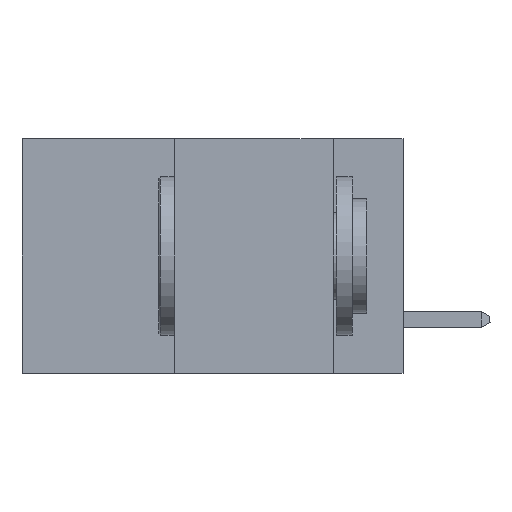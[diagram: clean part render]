
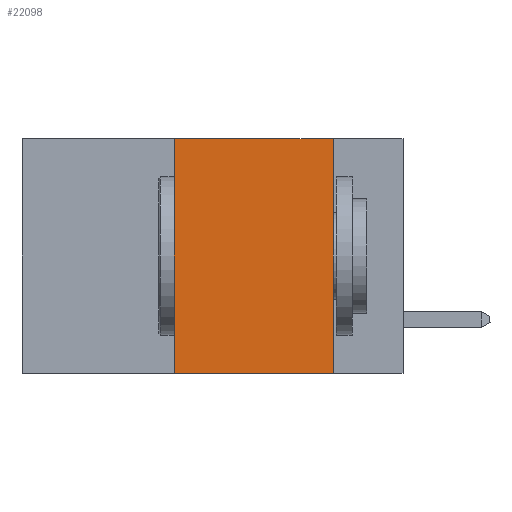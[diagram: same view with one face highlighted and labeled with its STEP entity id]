
A CAD part, left-side view. The second image highlights one B-rep face of the part: STEP entity #22098.
In plain terms, the highlighted planar face has unit normal (-1, 0, 0).
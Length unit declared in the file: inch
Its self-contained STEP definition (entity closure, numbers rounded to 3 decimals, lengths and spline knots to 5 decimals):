
#135 = ORIENTED_EDGE ( 'NONE', *, *, #2377, .T. ) ;
#674 = EDGE_CURVE ( 'NONE', #15671, #10634, #18919, .T. ) ;
#800 = EDGE_LOOP ( 'NONE', ( #26508, #30565, #5782, #135 ) ) ;
#1814 = DIRECTION ( 'NONE',  ( 0., -1., 0. ) ) ;
#1848 = CARTESIAN_POINT ( 'NONE',  ( 0., 0.6, -0.37 ) ) ;
#2271 = CARTESIAN_POINT ( 'NONE',  ( 0., 0.11, -0.37 ) ) ;
#2325 = VERTEX_POINT ( 'NONE', #2271 ) ;
#2377 = EDGE_CURVE ( 'NONE', #6501, #2325, #12804, .T. ) ;
#4229 = VECTOR ( 'NONE', #15766, 39.37008 ) ;
#5667 = EDGE_CURVE ( 'NONE', #6501, #15671, #22749, .T. ) ;
#5782 = ORIENTED_EDGE ( 'NONE', *, *, #5667, .F. ) ;
#6349 = PLANE ( 'NONE',  #23814 ) ;
#6501 = VERTEX_POINT ( 'NONE', #17493 ) ;
#6812 = VECTOR ( 'NONE', #27507, 39.37008 ) ;
#8775 = DIRECTION ( 'NONE',  ( 0., 0., -1. ) ) ;
#10634 = VERTEX_POINT ( 'NONE', #26943 ) ;
#11977 = CARTESIAN_POINT ( 'NONE',  ( 0., 0.36, 0. ) ) ;
#12068 = VECTOR ( 'NONE', #1814, 39.37008 ) ;
#12804 = LINE ( 'NONE', #1848, #12068 ) ;
#13348 = CARTESIAN_POINT ( 'NONE',  ( 0., 0.11, 0. ) ) ;
#15410 = EDGE_CURVE ( 'NONE', #10634, #2325, #23500, .T. ) ;
#15671 = VERTEX_POINT ( 'NONE', #21469 ) ;
#15766 = DIRECTION ( 'NONE',  ( 0., 0., -1. ) ) ;
#16331 = VECTOR ( 'NONE', #21680, 39.37008 ) ;
#17493 = CARTESIAN_POINT ( 'NONE',  ( 0., 0.36, -0.37 ) ) ;
#18919 = LINE ( 'NONE', #27606, #6812 ) ;
#20817 = CARTESIAN_POINT ( 'NONE',  ( 0., 0.6, 0. ) ) ;
#21469 = CARTESIAN_POINT ( 'NONE',  ( 0., 0.36, 0. ) ) ;
#21680 = DIRECTION ( 'NONE',  ( 0., 0., 1. ) ) ;
#22098 = ADVANCED_FACE ( 'NONE', ( #25140 ), #6349, .F. ) ;
#22749 = LINE ( 'NONE', #11977, #16331 ) ;
#23217 = DIRECTION ( 'NONE',  ( 1., 0., 0. ) ) ;
#23500 = LINE ( 'NONE', #13348, #4229 ) ;
#23814 = AXIS2_PLACEMENT_3D ( 'NONE', #20817, #23217, #8775 ) ;
#25140 = FACE_OUTER_BOUND ( 'NONE', #800, .T. ) ;
#26508 = ORIENTED_EDGE ( 'NONE', *, *, #15410, .F. ) ;
#26943 = CARTESIAN_POINT ( 'NONE',  ( 0., 0.11, 0. ) ) ;
#27507 = DIRECTION ( 'NONE',  ( 0., -1., 0. ) ) ;
#27606 = CARTESIAN_POINT ( 'NONE',  ( 0., 0.6, 0. ) ) ;
#30565 = ORIENTED_EDGE ( 'NONE', *, *, #674, .F. ) ;
